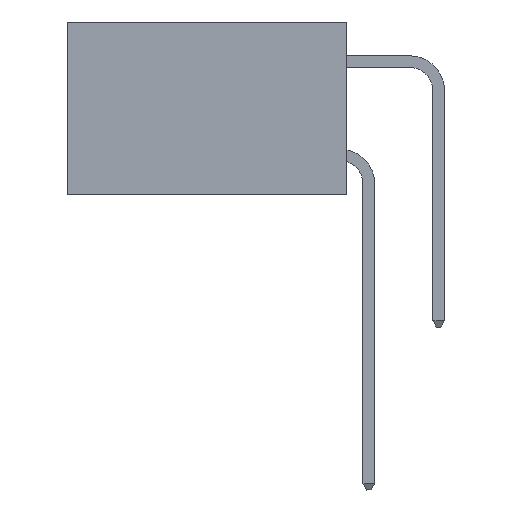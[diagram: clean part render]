
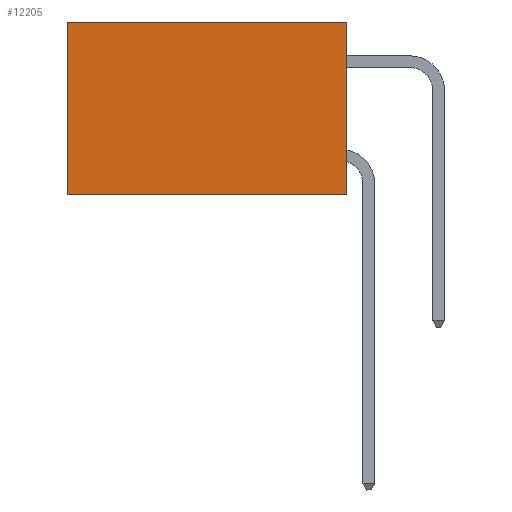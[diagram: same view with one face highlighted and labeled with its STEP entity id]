
A CAD part, left-side view. The second image highlights one B-rep face of the part: STEP entity #12205.
In plain terms, the highlighted planar face has unit normal (-1, 0, 0).
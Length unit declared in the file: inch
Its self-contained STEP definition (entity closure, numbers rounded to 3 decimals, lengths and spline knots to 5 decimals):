
#2576 = FACE_OUTER_BOUND ( 'NONE', #9567, .T. ) ;
#2593 = DIRECTION ( 'NONE',  ( 0., 1., 0. ) ) ;
#2685 = VECTOR ( 'NONE', #9228, 39.37008 ) ;
#3067 = AXIS2_PLACEMENT_3D ( 'NONE', #18342, #14118, #5156 ) ;
#3670 = VECTOR ( 'NONE', #2593, 39.37008 ) ;
#5039 = ORIENTED_EDGE ( 'NONE', *, *, #14726, .T. ) ;
#5156 = DIRECTION ( 'NONE',  ( 0., 0., -1. ) ) ;
#5952 = LINE ( 'NONE', #13195, #17662 ) ;
#7814 = LINE ( 'NONE', #9959, #3670 ) ;
#8006 = CARTESIAN_POINT ( 'NONE',  ( 0.2875, 0., -0.37 ) ) ;
#9228 = DIRECTION ( 'NONE',  ( 0., 1., 0. ) ) ;
#9567 = EDGE_LOOP ( 'NONE', ( #15478, #16927, #13713, #5039 ) ) ;
#9590 = EDGE_CURVE ( 'NONE', #10913, #16272, #11587, .T. ) ;
#9674 = PLANE ( 'NONE',  #3067 ) ;
#9959 = CARTESIAN_POINT ( 'NONE',  ( 0.2875, 0., 0. ) ) ;
#10702 = CARTESIAN_POINT ( 'NONE',  ( 0.2875, 0., -0.37 ) ) ;
#10913 = VERTEX_POINT ( 'NONE', #18453 ) ;
#11587 = LINE ( 'NONE', #16403, #18713 ) ;
#12205 = ADVANCED_FACE ( 'NONE', ( #2576 ), #9674, .F. ) ;
#13116 = CARTESIAN_POINT ( 'NONE',  ( 0.2875, 0.6, 0. ) ) ;
#13195 = CARTESIAN_POINT ( 'NONE',  ( 0.2875, 0.6, 0. ) ) ;
#13586 = EDGE_CURVE ( 'NONE', #16569, #17028, #5952, .T. ) ;
#13713 = ORIENTED_EDGE ( 'NONE', *, *, #9590, .F. ) ;
#14118 = DIRECTION ( 'NONE',  ( 1., 0., 0. ) ) ;
#14367 = EDGE_CURVE ( 'NONE', #16272, #17028, #18518, .T. ) ;
#14726 = EDGE_CURVE ( 'NONE', #10913, #16569, #7814, .T. ) ;
#14981 = DIRECTION ( 'NONE',  ( 0., 0., -1. ) ) ;
#15398 = CARTESIAN_POINT ( 'NONE',  ( 0.2875, 0.6, -0.37 ) ) ;
#15478 = ORIENTED_EDGE ( 'NONE', *, *, #13586, .T. ) ;
#16062 = DIRECTION ( 'NONE',  ( 0., 0., -1. ) ) ;
#16272 = VERTEX_POINT ( 'NONE', #8006 ) ;
#16403 = CARTESIAN_POINT ( 'NONE',  ( 0.2875, 0., 0. ) ) ;
#16569 = VERTEX_POINT ( 'NONE', #13116 ) ;
#16927 = ORIENTED_EDGE ( 'NONE', *, *, #14367, .F. ) ;
#17028 = VERTEX_POINT ( 'NONE', #15398 ) ;
#17662 = VECTOR ( 'NONE', #16062, 39.37008 ) ;
#18342 = CARTESIAN_POINT ( 'NONE',  ( 0.2875, 0., 0. ) ) ;
#18453 = CARTESIAN_POINT ( 'NONE',  ( 0.2875, 0., 0. ) ) ;
#18518 = LINE ( 'NONE', #10702, #2685 ) ;
#18713 = VECTOR ( 'NONE', #14981, 39.37008 ) ;
